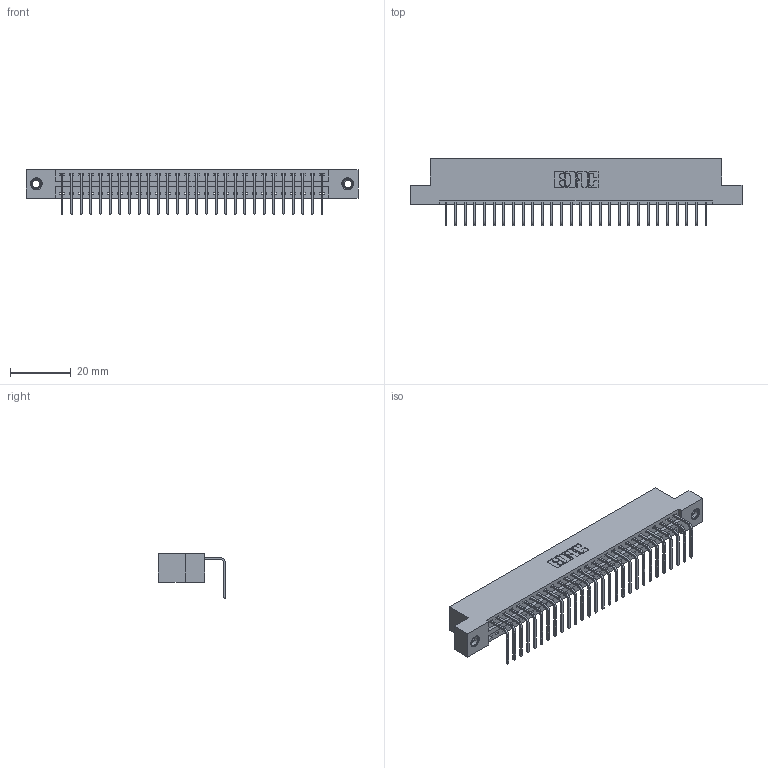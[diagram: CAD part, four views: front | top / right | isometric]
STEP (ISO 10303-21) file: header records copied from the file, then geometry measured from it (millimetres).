
FILE_DESCRIPTION (( 'STEP AP203' ), '1' );
FILE_NAME ('396-028-558-107.STEP', '2018-09-05T04:08:09', ( '' ), ( '' ), 'SwSTEP 2.0', 'SolidWorks 2016', '' );
FILE_SCHEMA (( 'CONFIG_CONTROL_DESIGN' ));
Length unit declared in the file: inch
Products named in the file (4): 346 Part_Flush Mounting Lugs - 0.156 Dia-TI; 345-292-001_558 Tail - 2; 345-250-001_345-250-005-103; 396-028-558-107
Assembly tree (31 placements, depth 2):
  396-028-558-107
    346 Part_Flush Mounting Lugs - 0.156 Dia-TI
    345-292-001_558 Tail - 2  x28
    345-250-001_345-250-005-103  x2
Bounding box: 109.47 x 22.16 x 14.73 mm (x, y, z)
Volume: 10462.4 mm3; surface area: 13516.8 mm2
Topology: 31 solids, 31 shells, 1862 faces, 5561 edges, 3662 vertices
Faces by surface type: plane 1284, cylinder 562, cone 12, torus 4
Entity records: 20532 total; most frequent: CARTESIAN_POINT 3507, ORIENTED_EDGE 3462, DIRECTION 3137, EDGE_CURVE 1731, VECTOR 1467, LINE 1467, VERTEX_POINT 1148, AXIS2_PLACEMENT_3D 835
